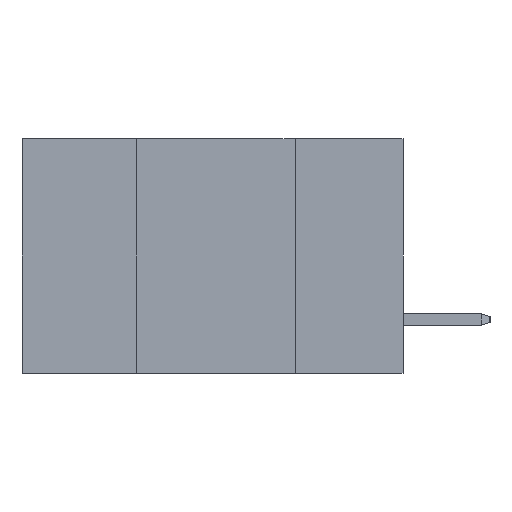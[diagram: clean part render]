
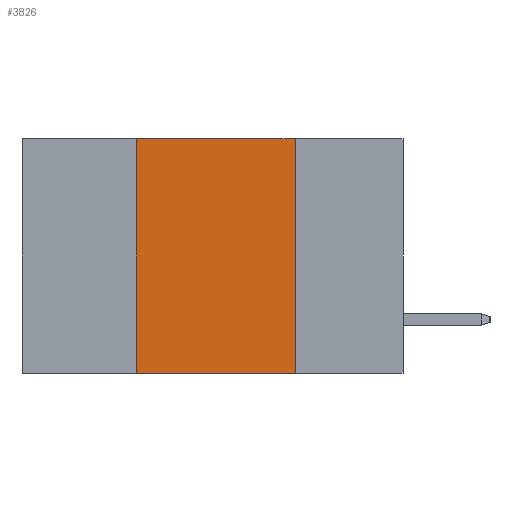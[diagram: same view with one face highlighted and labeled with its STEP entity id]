
A CAD part, left-side view. The second image highlights one B-rep face of the part: STEP entity #3826.
In plain terms, the highlighted planar face has unit normal (-1, 0, 0).
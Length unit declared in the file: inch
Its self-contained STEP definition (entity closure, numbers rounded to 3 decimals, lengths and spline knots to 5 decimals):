
#21 = EDGE_CURVE ( 'NONE', #14607, #4108, #7055, .T. ) ;
#23 = VECTOR ( 'NONE', #10776, 39.37008 ) ;
#731 = ORIENTED_EDGE ( 'NONE', *, *, #4965, .F. ) ;
#976 = LINE ( 'NONE', #2173, #23 ) ;
#1911 = EDGE_CURVE ( 'NONE', #15560, #15806, #15138, .T. ) ;
#2173 = CARTESIAN_POINT ( 'NONE',  ( 0., 0.42, 0. ) ) ;
#2480 = CARTESIAN_POINT ( 'NONE',  ( 0., 0.6, -0.37 ) ) ;
#3265 = ORIENTED_EDGE ( 'NONE', *, *, #21, .F. ) ;
#3826 = ADVANCED_FACE ( 'NONE', ( #8350 ), #10160, .F. ) ;
#4108 = VERTEX_POINT ( 'NONE', #9686 ) ;
#4576 = ORIENTED_EDGE ( 'NONE', *, *, #7732, .F. ) ;
#4965 = EDGE_CURVE ( 'NONE', #15560, #14607, #976, .T. ) ;
#5557 = VECTOR ( 'NONE', #8131, 39.37008 ) ;
#6172 = ORIENTED_EDGE ( 'NONE', *, *, #1911, .T. ) ;
#6316 = CARTESIAN_POINT ( 'NONE',  ( 0., 0.17, 0. ) ) ;
#6968 = CARTESIAN_POINT ( 'NONE',  ( 0., 0.17, -0.37 ) ) ;
#7055 = LINE ( 'NONE', #16986, #17273 ) ;
#7122 = CARTESIAN_POINT ( 'NONE',  ( 0., 0.42, 0. ) ) ;
#7732 = EDGE_CURVE ( 'NONE', #4108, #15806, #13110, .T. ) ;
#8131 = DIRECTION ( 'NONE',  ( 0., -1., 0. ) ) ;
#8350 = FACE_OUTER_BOUND ( 'NONE', #13004, .T. ) ;
#8789 = DIRECTION ( 'NONE',  ( 0., 0., -1. ) ) ;
#9480 = AXIS2_PLACEMENT_3D ( 'NONE', #12812, #13864, #14383 ) ;
#9686 = CARTESIAN_POINT ( 'NONE',  ( 0., 0.17, 0. ) ) ;
#10160 = PLANE ( 'NONE',  #9480 ) ;
#10776 = DIRECTION ( 'NONE',  ( 0., 0., 1. ) ) ;
#12812 = CARTESIAN_POINT ( 'NONE',  ( 0., 0.6, 0. ) ) ;
#13004 = EDGE_LOOP ( 'NONE', ( #4576, #3265, #731, #6172 ) ) ;
#13110 = LINE ( 'NONE', #6316, #17242 ) ;
#13854 = DIRECTION ( 'NONE',  ( 0., -1., 0. ) ) ;
#13864 = DIRECTION ( 'NONE',  ( 1., 0., 0. ) ) ;
#14383 = DIRECTION ( 'NONE',  ( 0., 0., -1. ) ) ;
#14607 = VERTEX_POINT ( 'NONE', #7122 ) ;
#15138 = LINE ( 'NONE', #2480, #5557 ) ;
#15560 = VERTEX_POINT ( 'NONE', #16186 ) ;
#15806 = VERTEX_POINT ( 'NONE', #6968 ) ;
#16186 = CARTESIAN_POINT ( 'NONE',  ( 0., 0.42, -0.37 ) ) ;
#16986 = CARTESIAN_POINT ( 'NONE',  ( 0., 0.6, 0. ) ) ;
#17242 = VECTOR ( 'NONE', #8789, 39.37008 ) ;
#17273 = VECTOR ( 'NONE', #13854, 39.37008 ) ;
